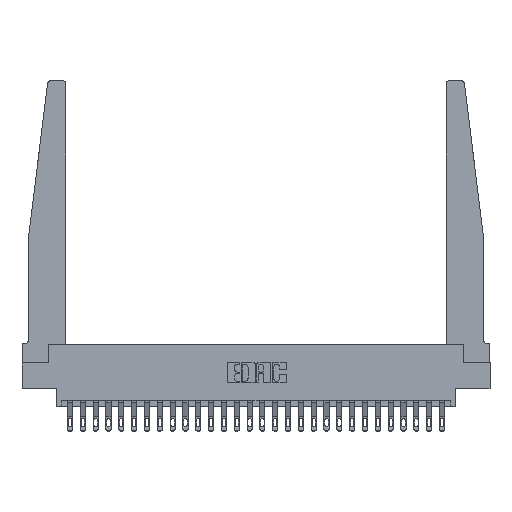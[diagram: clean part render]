
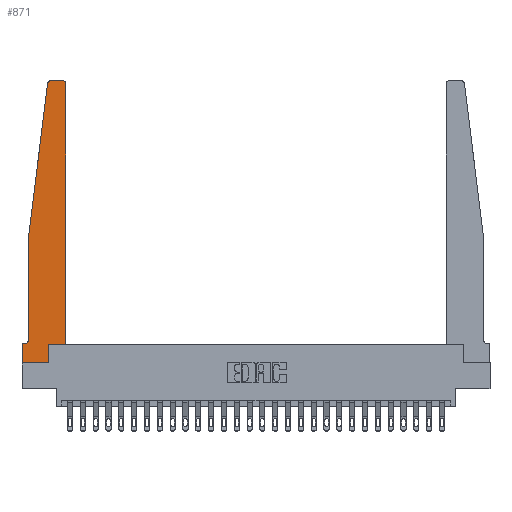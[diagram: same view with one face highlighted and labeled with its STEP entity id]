
A CAD part, top view. The second image highlights one B-rep face of the part: STEP entity #871.
In plain terms, the highlighted planar face has unit normal (0, 0, 1).
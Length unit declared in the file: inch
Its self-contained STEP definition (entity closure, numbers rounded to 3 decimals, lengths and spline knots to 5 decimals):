
#248 = ORIENTED_EDGE ( 'NONE', *, *, #20237, .T. ) ;
#308 = CARTESIAN_POINT ( 'NONE',  ( 0.27653, 2.75, 0.37 ) ) ;
#643 = DIRECTION ( 'NONE',  ( 1., 0., 0. ) ) ;
#871 = ADVANCED_FACE ( 'NONE', ( #4435 ), #6471, .T. ) ;
#1822 = VERTEX_POINT ( 'NONE', #17761 ) ;
#2357 = DIRECTION ( 'NONE',  ( 0., 0., -1. ) ) ;
#2709 = LINE ( 'NONE', #10966, #4808 ) ;
#3076 = LINE ( 'NONE', #11077, #7298 ) ;
#3200 = CARTESIAN_POINT ( 'NONE',  ( 0.27653, 2.72, 0.37 ) ) ;
#3344 = ORIENTED_EDGE ( 'NONE', *, *, #25360, .T. ) ;
#3372 = VERTEX_POINT ( 'NONE', #7850 ) ;
#3510 = EDGE_CURVE ( 'NONE', #3372, #6669, #13741, .T. ) ;
#3658 = EDGE_CURVE ( 'NONE', #19892, #17831, #3076, .T. ) ;
#3679 = DIRECTION ( 'NONE',  ( 0., -1., 0. ) ) ;
#4435 = FACE_OUTER_BOUND ( 'NONE', #16729, .T. ) ;
#4442 = DIRECTION ( 'NONE',  ( 1., 0., 0. ) ) ;
#4470 = CARTESIAN_POINT ( 'NONE',  ( 0., 0., 0.37 ) ) ;
#4808 = VECTOR ( 'NONE', #23771, 39.37008 ) ;
#4834 = EDGE_CURVE ( 'NONE', #1822, #19332, #6889, .T. ) ;
#6112 = ORIENTED_EDGE ( 'NONE', *, *, #4834, .T. ) ;
#6432 = CARTESIAN_POINT ( 'NONE',  ( 0.065, 0.2375, 0.37 ) ) ;
#6471 = PLANE ( 'NONE',  #14446 ) ;
#6551 = DIRECTION ( 'NONE',  ( -1., 0., 0. ) ) ;
#6648 = DIRECTION ( 'NONE',  ( 1., 0., 0. ) ) ;
#6669 = VERTEX_POINT ( 'NONE', #19379 ) ;
#6804 = DIRECTION ( 'NONE',  ( -1., 0., 0. ) ) ;
#6889 = LINE ( 'NONE', #21693, #11145 ) ;
#7298 = VECTOR ( 'NONE', #643, 39.37008 ) ;
#7549 = ORIENTED_EDGE ( 'NONE', *, *, #3510, .T. ) ;
#7583 = EDGE_CURVE ( 'NONE', #17831, #3372, #18564, .T. ) ;
#7850 = CARTESIAN_POINT ( 'NONE',  ( 0.425, 2.72, 0.37 ) ) ;
#7878 = CARTESIAN_POINT ( 'NONE',  ( 0.065, 1.25, 0.37 ) ) ;
#8239 = CARTESIAN_POINT ( 'NONE',  ( 0.395, 2.72, 0.37 ) ) ;
#8301 = EDGE_CURVE ( 'NONE', #15250, #12666, #9125, .T. ) ;
#8786 = ORIENTED_EDGE ( 'NONE', *, *, #7583, .T. ) ;
#8787 = CARTESIAN_POINT ( 'NONE',  ( 0.425, 0.18, 0.37 ) ) ;
#8827 = LINE ( 'NONE', #21738, #14522 ) ;
#9005 = AXIS2_PLACEMENT_3D ( 'NONE', #3200, #26438, #15657 ) ;
#9125 = CIRCLE ( 'NONE', #24324, 0.05 ) ;
#9230 = CARTESIAN_POINT ( 'NONE',  ( 0., 0.1875, 0.37 ) ) ;
#9416 = CARTESIAN_POINT ( 'NONE',  ( 0.2605, 0., 0.37 ) ) ;
#9841 = DIRECTION ( 'NONE',  ( 0., 1., 0. ) ) ;
#9862 = VERTEX_POINT ( 'NONE', #9416 ) ;
#9900 = LINE ( 'NONE', #7878, #21787 ) ;
#10396 = CARTESIAN_POINT ( 'NONE',  ( 0., 0.1875, 0.37 ) ) ;
#10966 = CARTESIAN_POINT ( 'NONE',  ( 0., 0., 0.37 ) ) ;
#11077 = CARTESIAN_POINT ( 'NONE',  ( 0.425, 0.18, 0.37 ) ) ;
#11145 = VECTOR ( 'NONE', #19792, 39.37008 ) ;
#12008 = CARTESIAN_POINT ( 'NONE',  ( 0.2605, 0.18, 0.37 ) ) ;
#12666 = VERTEX_POINT ( 'NONE', #23378 ) ;
#12785 = DIRECTION ( 'NONE',  ( -1., 0., 0. ) ) ;
#13741 = CIRCLE ( 'NONE', #14567, 0.03 ) ;
#13870 = VECTOR ( 'NONE', #25106, 39.37008 ) ;
#14415 = CARTESIAN_POINT ( 'NONE',  ( 0.015, 0.2375, 0.37 ) ) ;
#14446 = AXIS2_PLACEMENT_3D ( 'NONE', #10396, #17047, #16489 ) ;
#14522 = VECTOR ( 'NONE', #6804, 39.37008 ) ;
#14567 = AXIS2_PLACEMENT_3D ( 'NONE', #8239, #21151, #4442 ) ;
#14826 = ORIENTED_EDGE ( 'NONE', *, *, #18287, .T. ) ;
#15062 = ORIENTED_EDGE ( 'NONE', *, *, #24522, .T. ) ;
#15250 = VERTEX_POINT ( 'NONE', #6432 ) ;
#15657 = DIRECTION ( 'NONE',  ( 1., 0., 0. ) ) ;
#15951 = ORIENTED_EDGE ( 'NONE', *, *, #23741, .T. ) ;
#16049 = CARTESIAN_POINT ( 'NONE',  ( 0., 0., 0.37 ) ) ;
#16074 = EDGE_CURVE ( 'NONE', #6669, #23586, #8827, .T. ) ;
#16135 = ORIENTED_EDGE ( 'NONE', *, *, #3658, .T. ) ;
#16489 = DIRECTION ( 'NONE',  ( 1., 0., 0. ) ) ;
#16729 = EDGE_LOOP ( 'NONE', ( #20743, #14826, #6112, #3344, #26444, #248, #20802, #15951, #15062, #16135, #8786, #7549 ) ) ;
#17047 = DIRECTION ( 'NONE',  ( 0., 0., 1. ) ) ;
#17367 = VECTOR ( 'NONE', #6648, 39.37008 ) ;
#17761 = CARTESIAN_POINT ( 'NONE',  ( 0.24675, 2.72367, 0.37 ) ) ;
#17831 = VERTEX_POINT ( 'NONE', #21564 ) ;
#18287 = EDGE_CURVE ( 'NONE', #23586, #1822, #18961, .T. ) ;
#18326 = VERTEX_POINT ( 'NONE', #16049 ) ;
#18564 = LINE ( 'NONE', #8787, #13870 ) ;
#18859 = LINE ( 'NONE', #4470, #17367 ) ;
#18961 = CIRCLE ( 'NONE', #9005, 0.03 ) ;
#19332 = VERTEX_POINT ( 'NONE', #22246 ) ;
#19379 = CARTESIAN_POINT ( 'NONE',  ( 0.395, 2.75, 0.37 ) ) ;
#19468 = VECTOR ( 'NONE', #6551, 39.37008 ) ;
#19792 = DIRECTION ( 'NONE',  ( -0.122, -0.992, 0. ) ) ;
#19892 = VERTEX_POINT ( 'NONE', #26030 ) ;
#20237 = EDGE_CURVE ( 'NONE', #12666, #22058, #22730, .T. ) ;
#20445 = VECTOR ( 'NONE', #9841, 39.37008 ) ;
#20743 = ORIENTED_EDGE ( 'NONE', *, *, #16074, .T. ) ;
#20802 = ORIENTED_EDGE ( 'NONE', *, *, #23911, .T. ) ;
#21151 = DIRECTION ( 'NONE',  ( 0., 0., 1. ) ) ;
#21564 = CARTESIAN_POINT ( 'NONE',  ( 0.425, 0.18, 0.37 ) ) ;
#21693 = CARTESIAN_POINT ( 'NONE',  ( 0.065, 1.25, 0.37 ) ) ;
#21738 = CARTESIAN_POINT ( 'NONE',  ( 0.25, 2.75, 0.37 ) ) ;
#21787 = VECTOR ( 'NONE', #3679, 39.37008 ) ;
#22058 = VERTEX_POINT ( 'NONE', #9230 ) ;
#22246 = CARTESIAN_POINT ( 'NONE',  ( 0.065, 1.25, 0.37 ) ) ;
#22730 = LINE ( 'NONE', #24903, #19468 ) ;
#23378 = CARTESIAN_POINT ( 'NONE',  ( 0.015, 0.1875, 0.37 ) ) ;
#23586 = VERTEX_POINT ( 'NONE', #308 ) ;
#23741 = EDGE_CURVE ( 'NONE', #18326, #9862, #18859, .T. ) ;
#23771 = DIRECTION ( 'NONE',  ( 0., -1., 0. ) ) ;
#23911 = EDGE_CURVE ( 'NONE', #22058, #18326, #2709, .T. ) ;
#24324 = AXIS2_PLACEMENT_3D ( 'NONE', #14415, #2357, #12785 ) ;
#24522 = EDGE_CURVE ( 'NONE', #9862, #19892, #26841, .T. ) ;
#24903 = CARTESIAN_POINT ( 'NONE',  ( 0.065, 0.1875, 0.37 ) ) ;
#25106 = DIRECTION ( 'NONE',  ( 0., 1., 0. ) ) ;
#25360 = EDGE_CURVE ( 'NONE', #19332, #15250, #9900, .T. ) ;
#26030 = CARTESIAN_POINT ( 'NONE',  ( 0.2605, 0.18, 0.37 ) ) ;
#26438 = DIRECTION ( 'NONE',  ( 0., 0., 1. ) ) ;
#26444 = ORIENTED_EDGE ( 'NONE', *, *, #8301, .T. ) ;
#26841 = LINE ( 'NONE', #12008, #20445 ) ;
